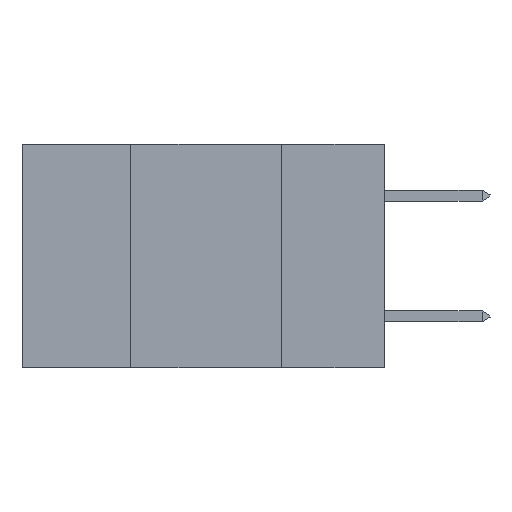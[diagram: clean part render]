
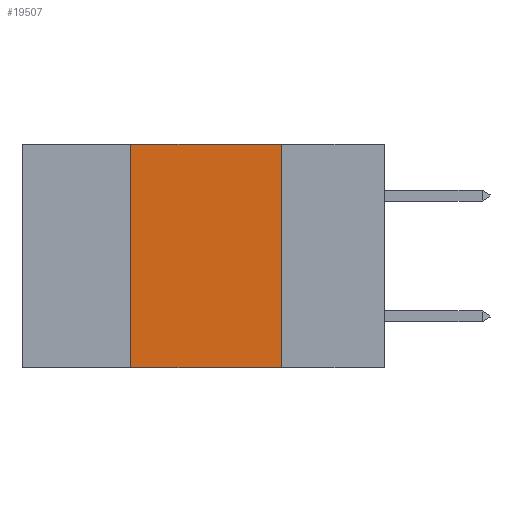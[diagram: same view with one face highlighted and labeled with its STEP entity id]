
A CAD part, left-side view. The second image highlights one B-rep face of the part: STEP entity #19507.
In plain terms, the highlighted planar face has unit normal (-1, 0, 0).
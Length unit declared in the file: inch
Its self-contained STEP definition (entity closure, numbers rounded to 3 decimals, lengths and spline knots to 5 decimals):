
#1592 = DIRECTION ( 'NONE',  ( 0., 0., 1. ) ) ;
#2449 = VERTEX_POINT ( 'NONE', #23182 ) ;
#2704 = ORIENTED_EDGE ( 'NONE', *, *, #25625, .T. ) ;
#3998 = CARTESIAN_POINT ( 'NONE',  ( 0., 0.6, 0. ) ) ;
#5608 = DIRECTION ( 'NONE',  ( 0., 0., -1. ) ) ;
#6286 = DIRECTION ( 'NONE',  ( 0., 0., -1. ) ) ;
#6364 = LINE ( 'NONE', #28060, #21341 ) ;
#8278 = AXIS2_PLACEMENT_3D ( 'NONE', #24546, #12299, #5608 ) ;
#8778 = VECTOR ( 'NONE', #16100, 39.37008 ) ;
#10432 = EDGE_LOOP ( 'NONE', ( #30901, #23792, #21420, #2704 ) ) ;
#11010 = VECTOR ( 'NONE', #1592, 39.37008 ) ;
#11785 = VECTOR ( 'NONE', #6286, 39.37008 ) ;
#12164 = LINE ( 'NONE', #20999, #11785 ) ;
#12299 = DIRECTION ( 'NONE',  ( 1., 0., 0. ) ) ;
#13089 = CARTESIAN_POINT ( 'NONE',  ( 0., 0.17, -0.37 ) ) ;
#15706 = LINE ( 'NONE', #3998, #8778 ) ;
#15810 = FACE_OUTER_BOUND ( 'NONE', #10432, .T. ) ;
#16100 = DIRECTION ( 'NONE',  ( 0., -1., 0. ) ) ;
#16946 = EDGE_CURVE ( 'NONE', #29705, #31461, #15706, .T. ) ;
#19055 = CARTESIAN_POINT ( 'NONE',  ( 0., 0.17, 0. ) ) ;
#19507 = ADVANCED_FACE ( 'NONE', ( #15810 ), #26881, .F. ) ;
#19530 = LINE ( 'NONE', #21754, #11010 ) ;
#20999 = CARTESIAN_POINT ( 'NONE',  ( 0., 0.17, 0. ) ) ;
#21170 = EDGE_CURVE ( 'NONE', #2449, #29705, #19530, .T. ) ;
#21341 = VECTOR ( 'NONE', #30460, 39.37008 ) ;
#21420 = ORIENTED_EDGE ( 'NONE', *, *, #21170, .F. ) ;
#21754 = CARTESIAN_POINT ( 'NONE',  ( 0., 0.42, 0. ) ) ;
#23182 = CARTESIAN_POINT ( 'NONE',  ( 0., 0.42, -0.37 ) ) ;
#23792 = ORIENTED_EDGE ( 'NONE', *, *, #16946, .F. ) ;
#24546 = CARTESIAN_POINT ( 'NONE',  ( 0., 0.6, 0. ) ) ;
#24744 = CARTESIAN_POINT ( 'NONE',  ( 0., 0.42, 0. ) ) ;
#25625 = EDGE_CURVE ( 'NONE', #2449, #27588, #6364, .T. ) ;
#26881 = PLANE ( 'NONE',  #8278 ) ;
#27588 = VERTEX_POINT ( 'NONE', #13089 ) ;
#28060 = CARTESIAN_POINT ( 'NONE',  ( 0., 0.6, -0.37 ) ) ;
#29705 = VERTEX_POINT ( 'NONE', #24744 ) ;
#30460 = DIRECTION ( 'NONE',  ( 0., -1., 0. ) ) ;
#30717 = EDGE_CURVE ( 'NONE', #31461, #27588, #12164, .T. ) ;
#30901 = ORIENTED_EDGE ( 'NONE', *, *, #30717, .F. ) ;
#31461 = VERTEX_POINT ( 'NONE', #19055 ) ;
